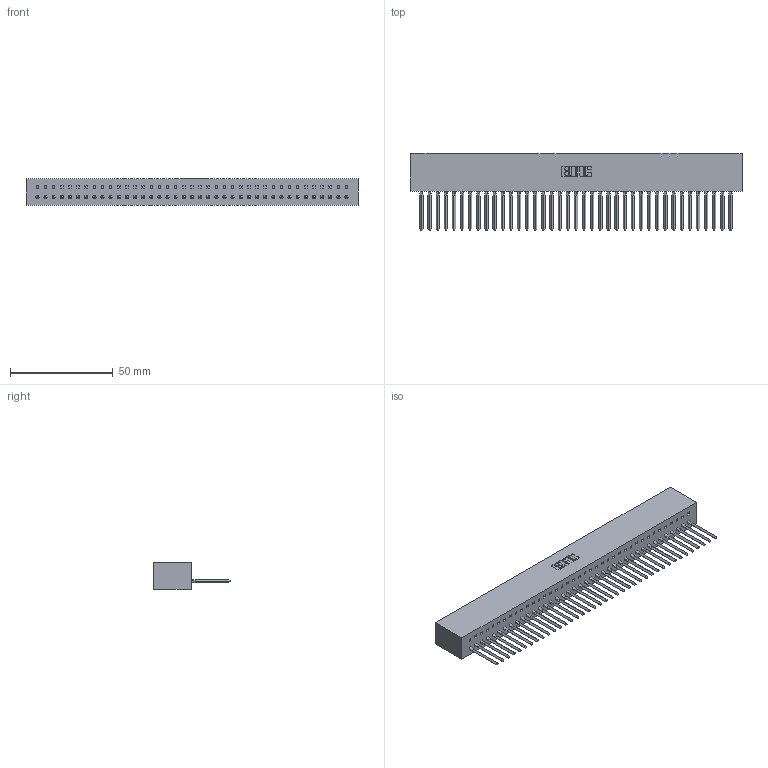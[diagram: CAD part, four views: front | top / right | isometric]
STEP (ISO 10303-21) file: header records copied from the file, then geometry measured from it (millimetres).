
FILE_DESCRIPTION (( 'STEP AP203' ), '1' );
FILE_NAME ('317-039-541-601.STEP', '2020-02-28T00:01:41', ( '' ), ( '' ), 'SwSTEP 2.0', 'SolidWorks 2016', '' );
FILE_SCHEMA (( 'CONFIG_CONTROL_DESIGN' ));
Length unit declared in the file: inch
Products named in the file (3): 317-290-002_541; 317-039-541-601; 317 Part_Lugless
Assembly tree (40 placements, depth 2):
  317-039-541-601
    317 Part_Lugless
    317-290-002_541  x39
Bounding box: 161.75 x 37.34 x 12.7 mm (x, y, z)
Volume: 27843.5 mm3; surface area: 39438.4 mm2
Topology: 40 solids, 40 shells, 6018 faces, 17165 edges, 11156 vertices
Faces by surface type: plane 4886, cylinder 976, bspline 156
Entity records: 56684 total; most frequent: CARTESIAN_POINT 10718, ORIENTED_EDGE 10010, DIRECTION 8211, EDGE_CURVE 5005, VECTOR 4649, LINE 4649, VERTEX_POINT 3328, AXIS2_PLACEMENT_3D 1781
